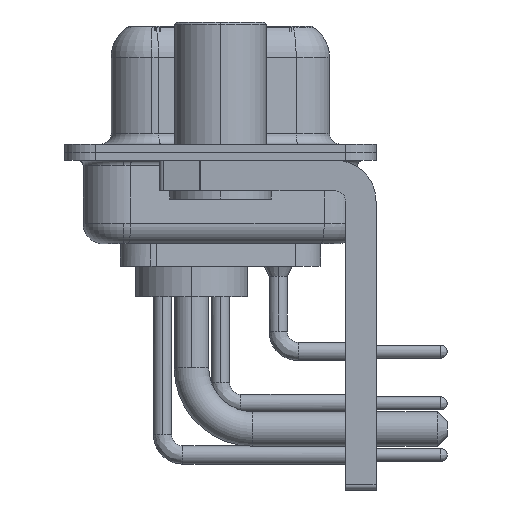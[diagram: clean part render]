
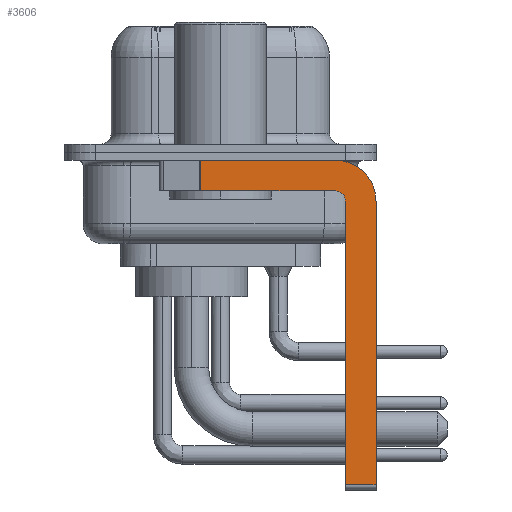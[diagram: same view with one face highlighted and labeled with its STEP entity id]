
A CAD part, left-side view. The second image highlights one B-rep face of the part: STEP entity #3606.
In plain terms, the highlighted planar face has unit normal (-1, 0, 0).
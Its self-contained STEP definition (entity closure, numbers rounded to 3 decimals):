
#327 = CARTESIAN_POINT ( 'NONE',  ( -2.9, -5.65, -2.4 ) ) ;
#518 = CARTESIAN_POINT ( 'NONE',  ( -2.9, -7.65, -2.4 ) ) ;
#1554 = LINE ( 'NONE', #12831, #11628 ) ;
#2105 = ORIENTED_EDGE ( 'NONE', *, *, #4943, .F. ) ;
#2497 = VERTEX_POINT ( 'NONE', #4120 ) ;
#2563 = PLANE ( 'NONE',  #36151 ) ;
#2717 = VECTOR ( 'NONE', #34059, 1000. ) ;
#2777 = VERTEX_POINT ( 'NONE', #5775 ) ;
#3606 = ADVANCED_FACE ( 'NONE', ( #14006 ), #2563, .F. ) ;
#4120 = CARTESIAN_POINT ( 'NONE',  ( -2.9, -7.65, -16.35 ) ) ;
#4190 = AXIS2_PLACEMENT_3D ( 'NONE', #9041, #14043, #22907 ) ;
#4881 = VECTOR ( 'NONE', #24421, 1000. ) ;
#4943 = EDGE_CURVE ( 'NONE', #2777, #2497, #14360, .T. ) ;
#5553 = CARTESIAN_POINT ( 'NONE',  ( -2.9, -5.65, -0.4 ) ) ;
#5775 = CARTESIAN_POINT ( 'NONE',  ( -2.9, -7.65, -2.4 ) ) ;
#6510 = ORIENTED_EDGE ( 'NONE', *, *, #16441, .T. ) ;
#7247 = VERTEX_POINT ( 'NONE', #5553 ) ;
#7551 = VECTOR ( 'NONE', #23292, 1000. ) ;
#8442 = EDGE_CURVE ( 'NONE', #14807, #2497, #1554, .T. ) ;
#8790 = VECTOR ( 'NONE', #21823, 1000. ) ;
#9041 = CARTESIAN_POINT ( 'NONE',  ( -2.9, -5.65, -2.4 ) ) ;
#9807 = ORIENTED_EDGE ( 'NONE', *, *, #15144, .F. ) ;
#10330 = EDGE_LOOP ( 'NONE', ( #34510, #6510, #18769, #33827, #24202, #35508, #2105, #9807 ) ) ;
#11615 = EDGE_CURVE ( 'NONE', #12286, #7247, #16841, .T. ) ;
#11628 = VECTOR ( 'NONE', #15955, 1000. ) ;
#12286 = VERTEX_POINT ( 'NONE', #20129 ) ;
#12831 = CARTESIAN_POINT ( 'NONE',  ( -2.9, -5.65, -16.35 ) ) ;
#13346 = VERTEX_POINT ( 'NONE', #24033 ) ;
#13528 = CARTESIAN_POINT ( 'NONE',  ( -2.9, 3., -0.4 ) ) ;
#14006 = FACE_OUTER_BOUND ( 'NONE', #10330, .T. ) ;
#14043 = DIRECTION ( 'NONE',  ( -1., 0., 0. ) ) ;
#14360 = LINE ( 'NONE', #518, #19066 ) ;
#14807 = VERTEX_POINT ( 'NONE', #32553 ) ;
#15118 = DIRECTION ( 'NONE',  ( 1., 0., 0. ) ) ;
#15144 = EDGE_CURVE ( 'NONE', #7247, #2777, #25263, .T. ) ;
#15295 = CARTESIAN_POINT ( 'NONE',  ( -2.9, -5.65, -2.4 ) ) ;
#15909 = CARTESIAN_POINT ( 'NONE',  ( -2.9, -6.15, -16.6 ) ) ;
#15955 = DIRECTION ( 'NONE',  ( 0., -1., 0. ) ) ;
#16441 = EDGE_CURVE ( 'NONE', #12286, #13346, #34513, .T. ) ;
#16841 = LINE ( 'NONE', #13528, #8790 ) ;
#18769 = ORIENTED_EDGE ( 'NONE', *, *, #25312, .F. ) ;
#19066 = VECTOR ( 'NONE', #22330, 1000. ) ;
#19515 = LINE ( 'NONE', #31132, #2717 ) ;
#19549 = DIRECTION ( 'NONE',  ( 0., 0., -1. ) ) ;
#19568 = EDGE_CURVE ( 'NONE', #20132, #30321, #33672, .T. ) ;
#19928 = AXIS2_PLACEMENT_3D ( 'NONE', #15295, #15118, #28491 ) ;
#20129 = CARTESIAN_POINT ( 'NONE',  ( -2.9, 0.978, -0.4 ) ) ;
#20132 = VERTEX_POINT ( 'NONE', #34624 ) ;
#21823 = DIRECTION ( 'NONE',  ( 0., -1., 0. ) ) ;
#22180 = EDGE_CURVE ( 'NONE', #14807, #20132, #32697, .T. ) ;
#22324 = DIRECTION ( 'NONE',  ( 1., 0., 0. ) ) ;
#22330 = DIRECTION ( 'NONE',  ( 0., 0., -1. ) ) ;
#22907 = DIRECTION ( 'NONE',  ( 0., 0., 1. ) ) ;
#23292 = DIRECTION ( 'NONE',  ( 0., 0., -1. ) ) ;
#24033 = CARTESIAN_POINT ( 'NONE',  ( -2.9, 0.978, -1.9 ) ) ;
#24202 = ORIENTED_EDGE ( 'NONE', *, *, #22180, .F. ) ;
#24421 = DIRECTION ( 'NONE',  ( 0., 0., 1. ) ) ;
#25263 = CIRCLE ( 'NONE', #19928, 2. ) ;
#25312 = EDGE_CURVE ( 'NONE', #30321, #13346, #19515, .T. ) ;
#28491 = DIRECTION ( 'NONE',  ( 0., 0., -1. ) ) ;
#28605 = CARTESIAN_POINT ( 'NONE',  ( -2.9, -5.65, -1.9 ) ) ;
#30321 = VERTEX_POINT ( 'NONE', #28605 ) ;
#31132 = CARTESIAN_POINT ( 'NONE',  ( -2.9, -5.65, -1.9 ) ) ;
#32553 = CARTESIAN_POINT ( 'NONE',  ( -2.9, -6.15, -16.35 ) ) ;
#32697 = LINE ( 'NONE', #15909, #4881 ) ;
#33672 = CIRCLE ( 'NONE', #4190, 0.5 ) ;
#33827 = ORIENTED_EDGE ( 'NONE', *, *, #19568, .F. ) ;
#34059 = DIRECTION ( 'NONE',  ( 0., 1., 0. ) ) ;
#34510 = ORIENTED_EDGE ( 'NONE', *, *, #11615, .F. ) ;
#34513 = LINE ( 'NONE', #34878, #7551 ) ;
#34624 = CARTESIAN_POINT ( 'NONE',  ( -2.9, -6.15, -2.4 ) ) ;
#34878 = CARTESIAN_POINT ( 'NONE',  ( -2.9, 0.978, -1.9 ) ) ;
#35508 = ORIENTED_EDGE ( 'NONE', *, *, #8442, .T. ) ;
#36151 = AXIS2_PLACEMENT_3D ( 'NONE', #327, #22324, #19549 ) ;
